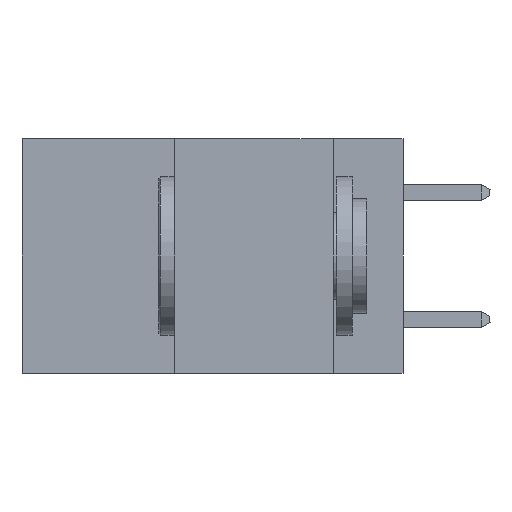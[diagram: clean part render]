
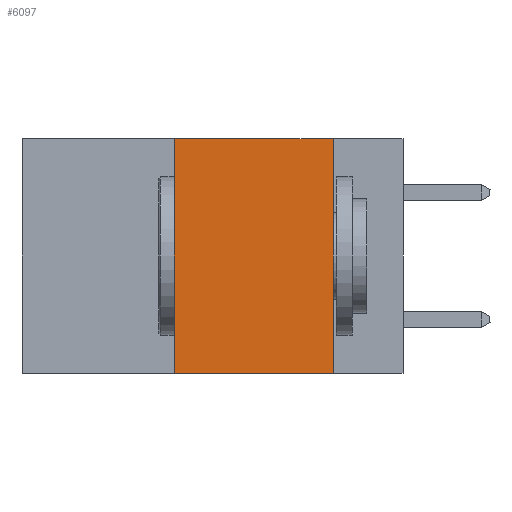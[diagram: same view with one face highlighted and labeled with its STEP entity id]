
A CAD part, left-side view. The second image highlights one B-rep face of the part: STEP entity #6097.
In plain terms, the highlighted planar face has unit normal (-1, 0, 0).
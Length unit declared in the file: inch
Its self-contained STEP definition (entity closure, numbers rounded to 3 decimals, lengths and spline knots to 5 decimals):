
#1281 = LINE ( 'NONE', #26277, #4159 ) ;
#1687 = CARTESIAN_POINT ( 'NONE',  ( 0., 0.11, -0.37 ) ) ;
#3429 = CARTESIAN_POINT ( 'NONE',  ( 0., 0.36, 0. ) ) ;
#4159 = VECTOR ( 'NONE', #18144, 39.37008 ) ;
#4209 = CARTESIAN_POINT ( 'NONE',  ( 0., 0.6, 0. ) ) ;
#4359 = EDGE_LOOP ( 'NONE', ( #23195, #17786, #12307, #9704 ) ) ;
#4959 = CARTESIAN_POINT ( 'NONE',  ( 0., 0.11, 0. ) ) ;
#6097 = ADVANCED_FACE ( 'NONE', ( #12335 ), #15418, .F. ) ;
#6806 = VERTEX_POINT ( 'NONE', #1687 ) ;
#7689 = VECTOR ( 'NONE', #26447, 39.37008 ) ;
#8719 = DIRECTION ( 'NONE',  ( 0., 0., -1. ) ) ;
#9704 = ORIENTED_EDGE ( 'NONE', *, *, #19404, .T. ) ;
#10002 = VECTOR ( 'NONE', #19299, 39.37008 ) ;
#10992 = VERTEX_POINT ( 'NONE', #22580 ) ;
#11081 = CARTESIAN_POINT ( 'NONE',  ( 0., 0.6, 0. ) ) ;
#11454 = DIRECTION ( 'NONE',  ( 0., 0., -1. ) ) ;
#12307 = ORIENTED_EDGE ( 'NONE', *, *, #21043, .F. ) ;
#12335 = FACE_OUTER_BOUND ( 'NONE', #4359, .T. ) ;
#12739 = VERTEX_POINT ( 'NONE', #13273 ) ;
#13273 = CARTESIAN_POINT ( 'NONE',  ( 0., 0.11, 0. ) ) ;
#14514 = LINE ( 'NONE', #23465, #10002 ) ;
#15418 = PLANE ( 'NONE',  #21045 ) ;
#15552 = LINE ( 'NONE', #4959, #26487 ) ;
#16753 = LINE ( 'NONE', #4209, #7689 ) ;
#17786 = ORIENTED_EDGE ( 'NONE', *, *, #20726, .F. ) ;
#18144 = DIRECTION ( 'NONE',  ( 0., 0., 1. ) ) ;
#18385 = EDGE_CURVE ( 'NONE', #12739, #6806, #15552, .T. ) ;
#19299 = DIRECTION ( 'NONE',  ( 0., -1., 0. ) ) ;
#19404 = EDGE_CURVE ( 'NONE', #10992, #6806, #14514, .T. ) ;
#20726 = EDGE_CURVE ( 'NONE', #26065, #12739, #16753, .T. ) ;
#21043 = EDGE_CURVE ( 'NONE', #10992, #26065, #1281, .T. ) ;
#21045 = AXIS2_PLACEMENT_3D ( 'NONE', #11081, #23939, #11454 ) ;
#22580 = CARTESIAN_POINT ( 'NONE',  ( 0., 0.36, -0.37 ) ) ;
#23195 = ORIENTED_EDGE ( 'NONE', *, *, #18385, .F. ) ;
#23465 = CARTESIAN_POINT ( 'NONE',  ( 0., 0.6, -0.37 ) ) ;
#23939 = DIRECTION ( 'NONE',  ( 1., 0., 0. ) ) ;
#26065 = VERTEX_POINT ( 'NONE', #3429 ) ;
#26277 = CARTESIAN_POINT ( 'NONE',  ( 0., 0.36, 0. ) ) ;
#26447 = DIRECTION ( 'NONE',  ( 0., -1., 0. ) ) ;
#26487 = VECTOR ( 'NONE', #8719, 39.37008 ) ;
